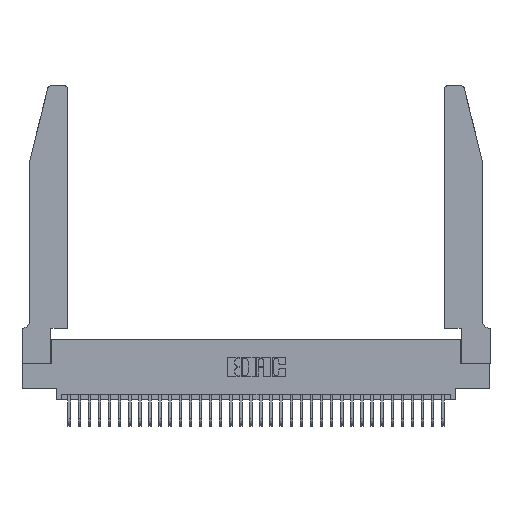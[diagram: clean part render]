
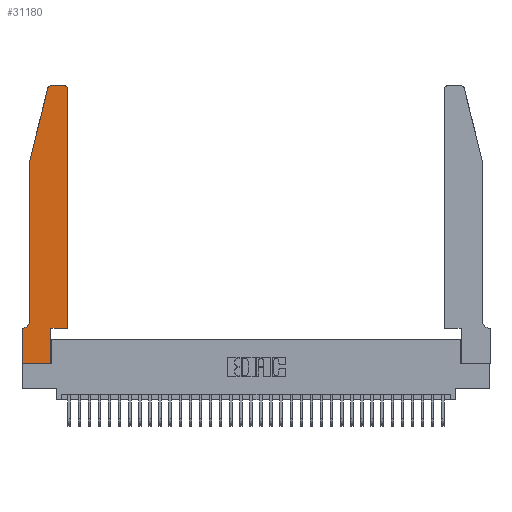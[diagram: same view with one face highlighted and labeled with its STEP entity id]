
A CAD part, top view. The second image highlights one B-rep face of the part: STEP entity #31180.
In plain terms, the highlighted planar face has unit normal (0, 0, 1).
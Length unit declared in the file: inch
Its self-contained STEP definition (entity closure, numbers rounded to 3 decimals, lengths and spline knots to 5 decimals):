
#245 = CARTESIAN_POINT ( 'NONE',  ( 0., 0.35, 0.37 ) ) ;
#342 = EDGE_LOOP ( 'NONE', ( #12187, #18103, #6205, #8825, #8721, #4501, #18628, #898, #4574, #15933, #18400, #14056 ) ) ;
#898 = ORIENTED_EDGE ( 'NONE', *, *, #13045, .T. ) ;
#1310 = VECTOR ( 'NONE', #3355, 39.37008 ) ;
#1662 = CIRCLE ( 'NONE', #22266, 0.03 ) ;
#2599 = CARTESIAN_POINT ( 'NONE',  ( 0.2605, 2.75, 0.37 ) ) ;
#2789 = CARTESIAN_POINT ( 'NONE',  ( 0.0755, 2., 0.37 ) ) ;
#2891 = CARTESIAN_POINT ( 'NONE',  ( 0.0755, 2., 0.37 ) ) ;
#3355 = DIRECTION ( 'NONE',  ( -1., 0., 0. ) ) ;
#3647 = CARTESIAN_POINT ( 'NONE',  ( 0.4505, 0.35, 0.37 ) ) ;
#3983 = CARTESIAN_POINT ( 'NONE',  ( 0.4505, 0.35, 0.37 ) ) ;
#4005 = CARTESIAN_POINT ( 'NONE',  ( 0.2865, 0.35, 0.37 ) ) ;
#4340 = VERTEX_POINT ( 'NONE', #2891 ) ;
#4501 = ORIENTED_EDGE ( 'NONE', *, *, #13198, .T. ) ;
#4574 = ORIENTED_EDGE ( 'NONE', *, *, #9423, .T. ) ;
#5070 = DIRECTION ( 'NONE',  ( 0., 0., -1. ) ) ;
#5519 = DIRECTION ( 'NONE',  ( -0.239, -0.971, 0. ) ) ;
#6205 = ORIENTED_EDGE ( 'NONE', *, *, #17392, .T. ) ;
#6382 = DIRECTION ( 'NONE',  ( 0., 1., 0. ) ) ;
#6496 = LINE ( 'NONE', #17205, #20547 ) ;
#6688 = DIRECTION ( 'NONE',  ( 0., -1., 0. ) ) ;
#6744 = DIRECTION ( 'NONE',  ( 0., 1., 0. ) ) ;
#6993 = VECTOR ( 'NONE', #6382, 39.37008 ) ;
#7307 = VECTOR ( 'NONE', #9819, 39.37008 ) ;
#7824 = CARTESIAN_POINT ( 'NONE',  ( 0., 0., 0.37 ) ) ;
#7882 = CARTESIAN_POINT ( 'NONE',  ( 0.0055, 0.35, 0.37 ) ) ;
#8014 = LINE ( 'NONE', #4005, #21208 ) ;
#8142 = LINE ( 'NONE', #17643, #7307 ) ;
#8581 = VERTEX_POINT ( 'NONE', #31795 ) ;
#8599 = VERTEX_POINT ( 'NONE', #245 ) ;
#8721 = ORIENTED_EDGE ( 'NONE', *, *, #26765, .T. ) ;
#8825 = ORIENTED_EDGE ( 'NONE', *, *, #23102, .T. ) ;
#9423 = EDGE_CURVE ( 'NONE', #24691, #33268, #8014, .T. ) ;
#9641 = VERTEX_POINT ( 'NONE', #7882 ) ;
#9682 = EDGE_CURVE ( 'NONE', #19332, #27260, #19971, .T. ) ;
#9819 = DIRECTION ( 'NONE',  ( 1., 0., 0. ) ) ;
#10051 = VERTEX_POINT ( 'NONE', #22591 ) ;
#10693 = CARTESIAN_POINT ( 'NONE',  ( 0., 0.35, 0.37 ) ) ;
#10794 = AXIS2_PLACEMENT_3D ( 'NONE', #20911, #5070, #23537 ) ;
#10906 = CIRCLE ( 'NONE', #10794, 0.07 ) ;
#11046 = FACE_OUTER_BOUND ( 'NONE', #342, .T. ) ;
#11521 = VECTOR ( 'NONE', #5519, 39.37008 ) ;
#11886 = CIRCLE ( 'NONE', #19172, 0.03 ) ;
#12187 = ORIENTED_EDGE ( 'NONE', *, *, #9682, .T. ) ;
#12682 = LINE ( 'NONE', #3983, #32676 ) ;
#13045 = EDGE_CURVE ( 'NONE', #10051, #24691, #8142, .T. ) ;
#13198 = EDGE_CURVE ( 'NONE', #9641, #8599, #22405, .T. ) ;
#13223 = CARTESIAN_POINT ( 'NONE',  ( 0.2865, 0., 0.37 ) ) ;
#13347 = DIRECTION ( 'NONE',  ( 1., 0., 0. ) ) ;
#13735 = CARTESIAN_POINT ( 'NONE',  ( 0.284, 2.72, 0.37 ) ) ;
#14056 = ORIENTED_EDGE ( 'NONE', *, *, #19951, .T. ) ;
#14619 = VECTOR ( 'NONE', #21251, 39.37008 ) ;
#15090 = CARTESIAN_POINT ( 'NONE',  ( 0.0755, 0.42, 0.37 ) ) ;
#15200 = CARTESIAN_POINT ( 'NONE',  ( 0.4205, 2.72, 0.37 ) ) ;
#15551 = VERTEX_POINT ( 'NONE', #15090 ) ;
#15660 = CARTESIAN_POINT ( 'NONE',  ( 0.0755, 0.35, 0.37 ) ) ;
#15933 = ORIENTED_EDGE ( 'NONE', *, *, #18903, .T. ) ;
#16374 = DIRECTION ( 'NONE',  ( 1., 0., 0. ) ) ;
#17205 = CARTESIAN_POINT ( 'NONE',  ( 0.0755, 2., 0.37 ) ) ;
#17392 = EDGE_CURVE ( 'NONE', #18506, #4340, #32366, .T. ) ;
#17643 = CARTESIAN_POINT ( 'NONE',  ( 0., 0., 0.37 ) ) ;
#17868 = DIRECTION ( 'NONE',  ( 1., 0., 0. ) ) ;
#18029 = EDGE_CURVE ( 'NONE', #27260, #18506, #11886, .T. ) ;
#18103 = ORIENTED_EDGE ( 'NONE', *, *, #18029, .T. ) ;
#18141 = VECTOR ( 'NONE', #28869, 39.37008 ) ;
#18400 = ORIENTED_EDGE ( 'NONE', *, *, #32438, .T. ) ;
#18506 = VERTEX_POINT ( 'NONE', #21266 ) ;
#18628 = ORIENTED_EDGE ( 'NONE', *, *, #29861, .T. ) ;
#18903 = EDGE_CURVE ( 'NONE', #33268, #8581, #12682, .T. ) ;
#19172 = AXIS2_PLACEMENT_3D ( 'NONE', #13735, #32011, #16374 ) ;
#19332 = VERTEX_POINT ( 'NONE', #19400 ) ;
#19400 = CARTESIAN_POINT ( 'NONE',  ( 0.4205, 2.75, 0.37 ) ) ;
#19951 = EDGE_CURVE ( 'NONE', #30922, #19332, #1662, .T. ) ;
#19971 = LINE ( 'NONE', #2599, #14619 ) ;
#20547 = VECTOR ( 'NONE', #6688, 39.37008 ) ;
#20911 = CARTESIAN_POINT ( 'NONE',  ( 0.0055, 0.42, 0.37 ) ) ;
#21208 = VECTOR ( 'NONE', #6744, 39.37008 ) ;
#21251 = DIRECTION ( 'NONE',  ( -1., 0., 0. ) ) ;
#21266 = CARTESIAN_POINT ( 'NONE',  ( 0.25487, 2.72718, 0.37 ) ) ;
#21630 = AXIS2_PLACEMENT_3D ( 'NONE', #10693, #29023, #13347 ) ;
#22266 = AXIS2_PLACEMENT_3D ( 'NONE', #15200, #33481, #17868 ) ;
#22405 = LINE ( 'NONE', #15660, #1310 ) ;
#22591 = CARTESIAN_POINT ( 'NONE',  ( 0., 0., 0.37 ) ) ;
#23102 = EDGE_CURVE ( 'NONE', #4340, #15551, #6496, .T. ) ;
#23537 = DIRECTION ( 'NONE',  ( -1., 0., 0. ) ) ;
#24691 = VERTEX_POINT ( 'NONE', #13223 ) ;
#25663 = CARTESIAN_POINT ( 'NONE',  ( 0.284, 2.75, 0.37 ) ) ;
#26376 = PLANE ( 'NONE',  #21630 ) ;
#26765 = EDGE_CURVE ( 'NONE', #15551, #9641, #10906, .T. ) ;
#27260 = VERTEX_POINT ( 'NONE', #25663 ) ;
#27772 = CARTESIAN_POINT ( 'NONE',  ( 0.4505, 2.72, 0.37 ) ) ;
#27977 = LINE ( 'NONE', #3647, #6993 ) ;
#28869 = DIRECTION ( 'NONE',  ( 0., -1., 0. ) ) ;
#29023 = DIRECTION ( 'NONE',  ( 0., 0., 1. ) ) ;
#29861 = EDGE_CURVE ( 'NONE', #8599, #10051, #32825, .T. ) ;
#30701 = CARTESIAN_POINT ( 'NONE',  ( 0.2865, 0.35, 0.37 ) ) ;
#30922 = VERTEX_POINT ( 'NONE', #27772 ) ;
#31180 = ADVANCED_FACE ( 'NONE', ( #11046 ), #26376, .T. ) ;
#31795 = CARTESIAN_POINT ( 'NONE',  ( 0.4505, 0.35, 0.37 ) ) ;
#32011 = DIRECTION ( 'NONE',  ( 0., 0., 1. ) ) ;
#32366 = LINE ( 'NONE', #2789, #11521 ) ;
#32438 = EDGE_CURVE ( 'NONE', #8581, #30922, #27977, .T. ) ;
#32676 = VECTOR ( 'NONE', #32990, 39.37008 ) ;
#32825 = LINE ( 'NONE', #7824, #18141 ) ;
#32990 = DIRECTION ( 'NONE',  ( 1., 0., 0. ) ) ;
#33268 = VERTEX_POINT ( 'NONE', #30701 ) ;
#33481 = DIRECTION ( 'NONE',  ( 0., 0., 1. ) ) ;
